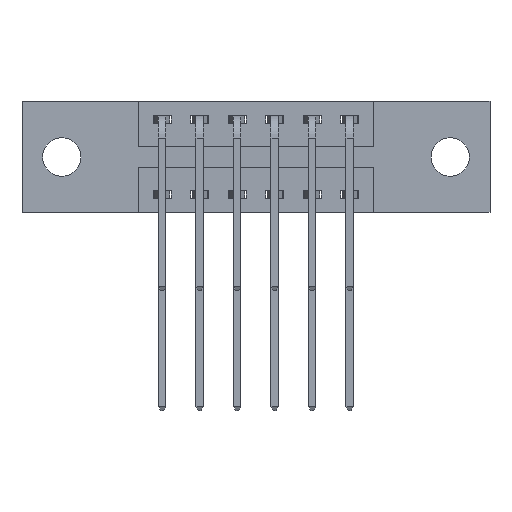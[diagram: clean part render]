
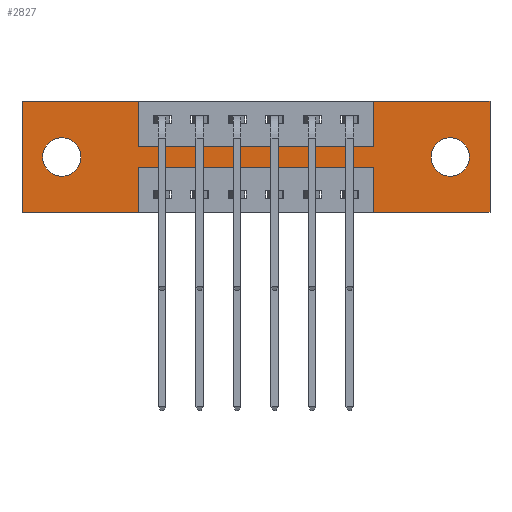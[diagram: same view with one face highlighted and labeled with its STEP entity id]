
A CAD part, front view. The second image highlights one B-rep face of the part: STEP entity #2827.
In plain terms, the highlighted planar face has unit normal (0, -1, 0).
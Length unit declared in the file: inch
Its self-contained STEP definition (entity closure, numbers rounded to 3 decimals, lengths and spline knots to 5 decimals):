
#173 = VERTEX_POINT ( 'NONE', #4392 ) ;
#260 = VERTEX_POINT ( 'NONE', #2740 ) ;
#331 = VECTOR ( 'NONE', #4372, 39.37008 ) ;
#709 = VERTEX_POINT ( 'NONE', #7489 ) ;
#730 = CIRCLE ( 'NONE', #7445, 0.064 ) ;
#736 = CARTESIAN_POINT ( 'NONE',  ( 0.1325, 0., -0.185 ) ) ;
#765 = FACE_OUTER_BOUND ( 'NONE', #2269, .T. ) ;
#769 = ORIENTED_EDGE ( 'NONE', *, *, #7471, .F. ) ;
#798 = EDGE_CURVE ( 'NONE', #10188, #1343, #7619, .T. ) ;
#881 = EDGE_CURVE ( 'NONE', #260, #2243, #6873, .T. ) ;
#994 = CIRCLE ( 'NONE', #7247, 0.064 ) ;
#1032 = EDGE_CURVE ( 'NONE', #3887, #3137, #3064, .T. ) ;
#1077 = DIRECTION ( 'NONE',  ( 1., 0., 0. ) ) ;
#1217 = CARTESIAN_POINT ( 'NONE',  ( 1.1725, 0., 0. ) ) ;
#1270 = DIRECTION ( 'NONE',  ( 0., -1., 0. ) ) ;
#1343 = VERTEX_POINT ( 'NONE', #3819 ) ;
#1388 = CARTESIAN_POINT ( 'NONE',  ( 1.4275, 0., -0.185 ) ) ;
#1461 = CARTESIAN_POINT ( 'NONE',  ( 1.1725, 0., -0.22 ) ) ;
#1569 = DIRECTION ( 'NONE',  ( 0., 0., 1. ) ) ;
#1712 = ORIENTED_EDGE ( 'NONE', *, *, #6966, .F. ) ;
#1781 = EDGE_LOOP ( 'NONE', ( #5926, #5813 ) ) ;
#1866 = CARTESIAN_POINT ( 'NONE',  ( 0.3875, 0., -0.15 ) ) ;
#1871 = DIRECTION ( 'NONE',  ( 0., 1., 0. ) ) ;
#1894 = CARTESIAN_POINT ( 'NONE',  ( 0.3875, 0., -0.22 ) ) ;
#1905 = LINE ( 'NONE', #2919, #6449 ) ;
#2011 = LINE ( 'NONE', #1866, #10446 ) ;
#2183 = ORIENTED_EDGE ( 'NONE', *, *, #7069, .F. ) ;
#2226 = DIRECTION ( 'NONE',  ( 0., 0., -1. ) ) ;
#2243 = VERTEX_POINT ( 'NONE', #3036 ) ;
#2269 = EDGE_LOOP ( 'NONE', ( #4084, #2693, #7981, #769, #2183, #9463, #4308, #2520, #6110, #3967, #1712, #9696 ) ) ;
#2431 = CARTESIAN_POINT ( 'NONE',  ( 1.1725, 0., 0. ) ) ;
#2458 = VECTOR ( 'NONE', #5341, 39.37008 ) ;
#2520 = ORIENTED_EDGE ( 'NONE', *, *, #10445, .F. ) ;
#2683 = DIRECTION ( 'NONE',  ( 0., 0., 1. ) ) ;
#2693 = ORIENTED_EDGE ( 'NONE', *, *, #9149, .F. ) ;
#2740 = CARTESIAN_POINT ( 'NONE',  ( 0., 0., 0. ) ) ;
#2768 = VERTEX_POINT ( 'NONE', #7795 ) ;
#2803 = AXIS2_PLACEMENT_3D ( 'NONE', #4558, #1871, #3607 ) ;
#2807 = CARTESIAN_POINT ( 'NONE',  ( 1.56, 0., 0. ) ) ;
#2827 = ADVANCED_FACE ( 'NONE', ( #5533, #9333, #765 ), #6377, .T. ) ;
#2870 = LINE ( 'NONE', #1217, #7028 ) ;
#2919 = CARTESIAN_POINT ( 'NONE',  ( 0., 0., -0.37 ) ) ;
#2921 = CARTESIAN_POINT ( 'NONE',  ( 1.1725, 0., -0.37 ) ) ;
#3036 = CARTESIAN_POINT ( 'NONE',  ( 0.3875, 0., 0. ) ) ;
#3051 = EDGE_LOOP ( 'NONE', ( #9199, #10161 ) ) ;
#3064 = LINE ( 'NONE', #5088, #9362 ) ;
#3137 = VERTEX_POINT ( 'NONE', #7505 ) ;
#3508 = VECTOR ( 'NONE', #5915, 39.37008 ) ;
#3512 = VERTEX_POINT ( 'NONE', #5367 ) ;
#3515 = CARTESIAN_POINT ( 'NONE',  ( 0.3875, 0., 0. ) ) ;
#3529 = CARTESIAN_POINT ( 'NONE',  ( 0.3875, 0., -0.22 ) ) ;
#3607 = DIRECTION ( 'NONE',  ( 0., 0., 1. ) ) ;
#3756 = LINE ( 'NONE', #9884, #3508 ) ;
#3819 = CARTESIAN_POINT ( 'NONE',  ( 0.1325, 0., -0.121 ) ) ;
#3852 = AXIS2_PLACEMENT_3D ( 'NONE', #5509, #1270, #7151 ) ;
#3887 = VERTEX_POINT ( 'NONE', #2431 ) ;
#3967 = ORIENTED_EDGE ( 'NONE', *, *, #881, .F. ) ;
#4084 = ORIENTED_EDGE ( 'NONE', *, *, #8949, .F. ) ;
#4262 = EDGE_CURVE ( 'NONE', #709, #6311, #730, .T. ) ;
#4308 = ORIENTED_EDGE ( 'NONE', *, *, #9538, .F. ) ;
#4372 = DIRECTION ( 'NONE',  ( 0., 0., -1. ) ) ;
#4392 = CARTESIAN_POINT ( 'NONE',  ( 1.1725, 0., -0.37 ) ) ;
#4558 = CARTESIAN_POINT ( 'NONE',  ( 0.1325, 0., -0.185 ) ) ;
#4674 = CARTESIAN_POINT ( 'NONE',  ( 1.4275, 0., -0.185 ) ) ;
#4716 = VECTOR ( 'NONE', #7704, 39.37008 ) ;
#5055 = VERTEX_POINT ( 'NONE', #1894 ) ;
#5088 = CARTESIAN_POINT ( 'NONE',  ( 0., 0., 0. ) ) ;
#5111 = VECTOR ( 'NONE', #10213, 39.37008 ) ;
#5341 = DIRECTION ( 'NONE',  ( 0., 0., -1. ) ) ;
#5367 = CARTESIAN_POINT ( 'NONE',  ( 1.1725, 0., -0.15 ) ) ;
#5509 = CARTESIAN_POINT ( 'NONE',  ( 0., 0., -0.37 ) ) ;
#5516 = DIRECTION ( 'NONE',  ( 0., 0., -1. ) ) ;
#5529 = LINE ( 'NONE', #6864, #7705 ) ;
#5533 = FACE_BOUND ( 'NONE', #3051, .T. ) ;
#5813 = ORIENTED_EDGE ( 'NONE', *, *, #798, .T. ) ;
#5840 = AXIS2_PLACEMENT_3D ( 'NONE', #4674, #10267, #5516 ) ;
#5915 = DIRECTION ( 'NONE',  ( 0., 0., -1. ) ) ;
#5926 = ORIENTED_EDGE ( 'NONE', *, *, #8226, .T. ) ;
#6018 = CARTESIAN_POINT ( 'NONE',  ( 1.4275, 0., -0.121 ) ) ;
#6098 = DIRECTION ( 'NONE',  ( -1., 0., 0. ) ) ;
#6110 = ORIENTED_EDGE ( 'NONE', *, *, #10321, .F. ) ;
#6235 = DIRECTION ( 'NONE',  ( 1., 0., 0. ) ) ;
#6311 = VERTEX_POINT ( 'NONE', #6018 ) ;
#6318 = DIRECTION ( 'NONE',  ( 0., 0., 1. ) ) ;
#6377 = PLANE ( 'NONE',  #3852 ) ;
#6442 = CARTESIAN_POINT ( 'NONE',  ( 0.3875, 0., -0.15 ) ) ;
#6449 = VECTOR ( 'NONE', #10181, 39.37008 ) ;
#6642 = VERTEX_POINT ( 'NONE', #1461 ) ;
#6659 = DIRECTION ( 'NONE',  ( 0., 1., 0. ) ) ;
#6864 = CARTESIAN_POINT ( 'NONE',  ( 0., 0., 0. ) ) ;
#6873 = LINE ( 'NONE', #8911, #9253 ) ;
#6966 = EDGE_CURVE ( 'NONE', #7997, #260, #5529, .T. ) ;
#7022 = LINE ( 'NONE', #3515, #331 ) ;
#7028 = VECTOR ( 'NONE', #6318, 39.37008 ) ;
#7069 = EDGE_CURVE ( 'NONE', #3137, #8126, #8870, .T. ) ;
#7151 = DIRECTION ( 'NONE',  ( 0., 0., -1. ) ) ;
#7247 = AXIS2_PLACEMENT_3D ( 'NONE', #736, #6659, #1569 ) ;
#7262 = DIRECTION ( 'NONE',  ( 0., 1., 0. ) ) ;
#7295 = VERTEX_POINT ( 'NONE', #6442 ) ;
#7445 = AXIS2_PLACEMENT_3D ( 'NONE', #1388, #7262, #2226 ) ;
#7471 = EDGE_CURVE ( 'NONE', #8126, #173, #1905, .T. ) ;
#7489 = CARTESIAN_POINT ( 'NONE',  ( 1.4275, 0., -0.249 ) ) ;
#7505 = CARTESIAN_POINT ( 'NONE',  ( 1.56, 0., 0. ) ) ;
#7619 = CIRCLE ( 'NONE', #2803, 0.064 ) ;
#7704 = DIRECTION ( 'NONE',  ( -1., 0., 0. ) ) ;
#7705 = VECTOR ( 'NONE', #2683, 39.37008 ) ;
#7795 = CARTESIAN_POINT ( 'NONE',  ( 0.3875, 0., -0.37 ) ) ;
#7820 = EDGE_CURVE ( 'NONE', #2768, #7997, #9307, .T. ) ;
#7981 = ORIENTED_EDGE ( 'NONE', *, *, #9512, .F. ) ;
#7997 = VERTEX_POINT ( 'NONE', #9376 ) ;
#8048 = EDGE_CURVE ( 'NONE', #6311, #709, #9181, .T. ) ;
#8126 = VERTEX_POINT ( 'NONE', #10411 ) ;
#8226 = EDGE_CURVE ( 'NONE', #1343, #10188, #994, .T. ) ;
#8504 = CARTESIAN_POINT ( 'NONE',  ( 0., 0., -0.37 ) ) ;
#8837 = VECTOR ( 'NONE', #6098, 39.37008 ) ;
#8870 = LINE ( 'NONE', #2807, #2458 ) ;
#8911 = CARTESIAN_POINT ( 'NONE',  ( 0., 0., 0. ) ) ;
#8949 = EDGE_CURVE ( 'NONE', #5055, #2768, #3756, .T. ) ;
#9064 = LINE ( 'NONE', #3529, #8837 ) ;
#9149 = EDGE_CURVE ( 'NONE', #6642, #5055, #9064, .T. ) ;
#9181 = CIRCLE ( 'NONE', #5840, 0.064 ) ;
#9199 = ORIENTED_EDGE ( 'NONE', *, *, #8048, .T. ) ;
#9253 = VECTOR ( 'NONE', #6235, 39.37008 ) ;
#9307 = LINE ( 'NONE', #8504, #4716 ) ;
#9333 = FACE_BOUND ( 'NONE', #1781, .T. ) ;
#9344 = DIRECTION ( 'NONE',  ( 1., 0., 0. ) ) ;
#9362 = VECTOR ( 'NONE', #1077, 39.37008 ) ;
#9376 = CARTESIAN_POINT ( 'NONE',  ( 0., 0., -0.37 ) ) ;
#9409 = LINE ( 'NONE', #2921, #5111 ) ;
#9463 = ORIENTED_EDGE ( 'NONE', *, *, #1032, .F. ) ;
#9512 = EDGE_CURVE ( 'NONE', #173, #6642, #9409, .T. ) ;
#9538 = EDGE_CURVE ( 'NONE', #3512, #3887, #2870, .T. ) ;
#9696 = ORIENTED_EDGE ( 'NONE', *, *, #7820, .F. ) ;
#9871 = CARTESIAN_POINT ( 'NONE',  ( 0.1325, 0., -0.249 ) ) ;
#9884 = CARTESIAN_POINT ( 'NONE',  ( 0.3875, 0., -0.37 ) ) ;
#10161 = ORIENTED_EDGE ( 'NONE', *, *, #4262, .T. ) ;
#10181 = DIRECTION ( 'NONE',  ( -1., 0., 0. ) ) ;
#10188 = VERTEX_POINT ( 'NONE', #9871 ) ;
#10213 = DIRECTION ( 'NONE',  ( 0., 0., 1. ) ) ;
#10267 = DIRECTION ( 'NONE',  ( 0., 1., 0. ) ) ;
#10321 = EDGE_CURVE ( 'NONE', #2243, #7295, #7022, .T. ) ;
#10411 = CARTESIAN_POINT ( 'NONE',  ( 1.56, 0., -0.37 ) ) ;
#10445 = EDGE_CURVE ( 'NONE', #7295, #3512, #2011, .T. ) ;
#10446 = VECTOR ( 'NONE', #9344, 39.37008 ) ;
